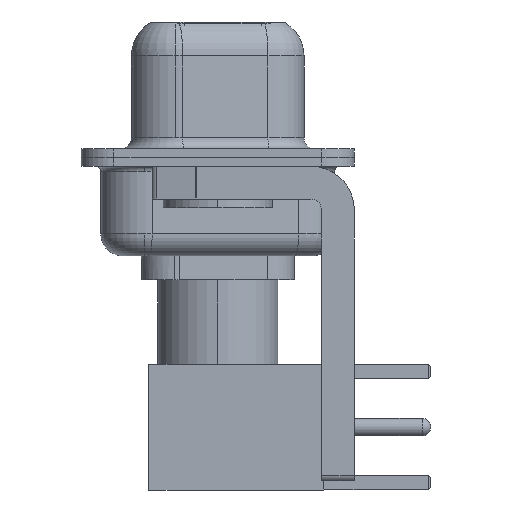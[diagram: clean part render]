
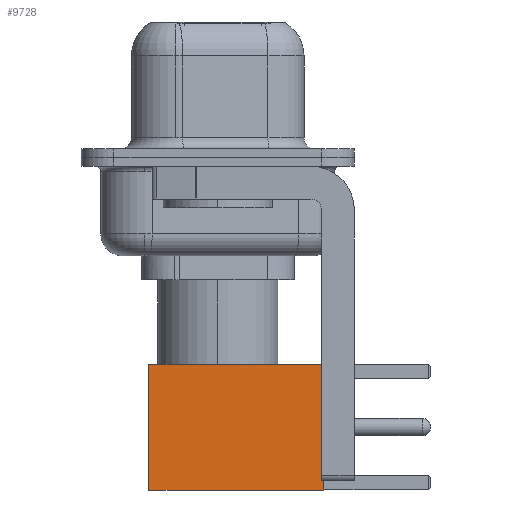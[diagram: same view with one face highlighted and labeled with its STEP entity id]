
A CAD part, left-side view. The second image highlights one B-rep face of the part: STEP entity #9728.
In plain terms, the highlighted face is planar.
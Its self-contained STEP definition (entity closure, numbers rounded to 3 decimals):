
#164 = EDGE_CURVE ( 'NONE', #1205, #2108, #5007, .T. ) ;
#725 = VECTOR ( 'NONE', #10871, 1000. ) ;
#1149 = EDGE_CURVE ( 'NONE', #1368, #1205, #2388, .T. ) ;
#1205 = VERTEX_POINT ( 'NONE', #13171 ) ;
#1368 = VERTEX_POINT ( 'NONE', #3405 ) ;
#1865 = LINE ( 'NONE', #9425, #6432 ) ;
#2108 = VERTEX_POINT ( 'NONE', #6165 ) ;
#2334 = DIRECTION ( 'NONE',  ( 0., 1., 0. ) ) ;
#2388 = LINE ( 'NONE', #14117, #725 ) ;
#2586 = DIRECTION ( 'NONE',  ( 0., 0., -1. ) ) ;
#3405 = CARTESIAN_POINT ( 'NONE',  ( 2.875, 2.875, 8. ) ) ;
#3934 = EDGE_LOOP ( 'NONE', ( #8972, #14741, #13350, #16628 ) ) ;
#4979 = FACE_OUTER_BOUND ( 'NONE', #3934, .T. ) ;
#5007 = LINE ( 'NONE', #12652, #7789 ) ;
#6165 = CARTESIAN_POINT ( 'NONE',  ( -2.875, 2.875, 0. ) ) ;
#6316 = PLANE ( 'NONE',  #8214 ) ;
#6432 = VECTOR ( 'NONE', #14618, 1000. ) ;
#7789 = VECTOR ( 'NONE', #14004, 1000. ) ;
#8214 = AXIS2_PLACEMENT_3D ( 'NONE', #13984, #2334, #11510 ) ;
#8972 = ORIENTED_EDGE ( 'NONE', *, *, #9088, .T. ) ;
#9088 = EDGE_CURVE ( 'NONE', #1368, #15861, #9725, .T. ) ;
#9425 = CARTESIAN_POINT ( 'NONE',  ( 0., 2.875, 0. ) ) ;
#9725 = LINE ( 'NONE', #14913, #12322 ) ;
#9728 = ADVANCED_FACE ( 'NONE', ( #4979 ), #6316, .T. ) ;
#10442 = CARTESIAN_POINT ( 'NONE',  ( 2.875, 2.875, 0. ) ) ;
#10871 = DIRECTION ( 'NONE',  ( -1., 0., 0. ) ) ;
#11510 = DIRECTION ( 'NONE',  ( 0., 0., 1. ) ) ;
#12322 = VECTOR ( 'NONE', #2586, 1000. ) ;
#12652 = CARTESIAN_POINT ( 'NONE',  ( -2.875, 2.875, 0. ) ) ;
#13171 = CARTESIAN_POINT ( 'NONE',  ( -2.875, 2.875, 8. ) ) ;
#13350 = ORIENTED_EDGE ( 'NONE', *, *, #164, .F. ) ;
#13984 = CARTESIAN_POINT ( 'NONE',  ( 2.875, 2.875, 0. ) ) ;
#14004 = DIRECTION ( 'NONE',  ( 0., 0., -1. ) ) ;
#14117 = CARTESIAN_POINT ( 'NONE',  ( 0., 2.875, 8. ) ) ;
#14608 = EDGE_CURVE ( 'NONE', #15861, #2108, #1865, .T. ) ;
#14618 = DIRECTION ( 'NONE',  ( -1., 0., 0. ) ) ;
#14741 = ORIENTED_EDGE ( 'NONE', *, *, #14608, .T. ) ;
#14913 = CARTESIAN_POINT ( 'NONE',  ( 2.875, 2.875, 0. ) ) ;
#15861 = VERTEX_POINT ( 'NONE', #10442 ) ;
#16628 = ORIENTED_EDGE ( 'NONE', *, *, #1149, .F. ) ;
